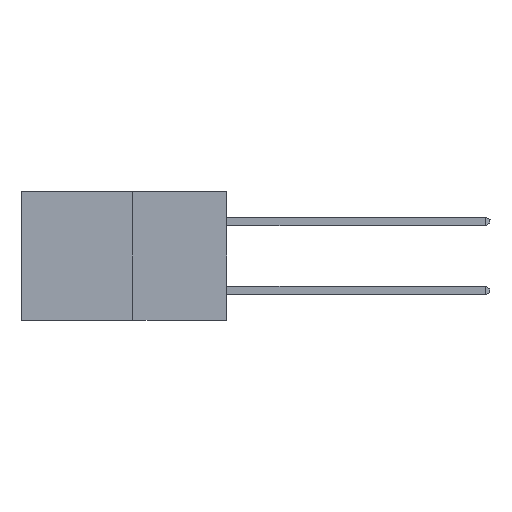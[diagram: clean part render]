
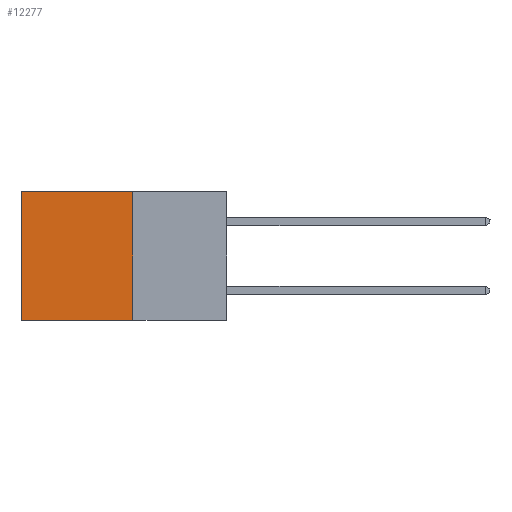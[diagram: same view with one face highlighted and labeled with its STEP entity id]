
A CAD part, left-side view. The second image highlights one B-rep face of the part: STEP entity #12277.
In plain terms, the highlighted planar face has unit normal (-1, 0, 0).
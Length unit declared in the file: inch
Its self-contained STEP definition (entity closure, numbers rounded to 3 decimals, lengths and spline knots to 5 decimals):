
#582 = EDGE_LOOP ( 'NONE', ( #15951, #666, #16527, #18513 ) ) ;
#633 = VERTEX_POINT ( 'NONE', #894 ) ;
#666 = ORIENTED_EDGE ( 'NONE', *, *, #5503, .F. ) ;
#894 = CARTESIAN_POINT ( 'NONE',  ( 0.277, 0.27, -0.37 ) ) ;
#1776 = EDGE_CURVE ( 'NONE', #5112, #1780, #6672, .T. ) ;
#1780 = VERTEX_POINT ( 'NONE', #5195 ) ;
#2743 = EDGE_CURVE ( 'NONE', #3079, #633, #12970, .T. ) ;
#3079 = VERTEX_POINT ( 'NONE', #8155 ) ;
#3580 = CARTESIAN_POINT ( 'NONE',  ( 0.277, 0.59, -0.37 ) ) ;
#3604 = DIRECTION ( 'NONE',  ( 0., 0., -1. ) ) ;
#5112 = VERTEX_POINT ( 'NONE', #13423 ) ;
#5195 = CARTESIAN_POINT ( 'NONE',  ( 0.277, 0.59, -0.37 ) ) ;
#5503 = EDGE_CURVE ( 'NONE', #633, #1780, #16423, .T. ) ;
#6672 = LINE ( 'NONE', #3580, #18489 ) ;
#7675 = CARTESIAN_POINT ( 'NONE',  ( 0.277, 0.27, -0.37 ) ) ;
#7895 = VECTOR ( 'NONE', #17598, 39.37008 ) ;
#8155 = CARTESIAN_POINT ( 'NONE',  ( 0.277, 0.27, 0. ) ) ;
#9320 = DIRECTION ( 'NONE',  ( 1., 0., 0. ) ) ;
#9651 = CARTESIAN_POINT ( 'NONE',  ( 0.277, 0.27, -0.37 ) ) ;
#10690 = LINE ( 'NONE', #20154, #19179 ) ;
#12277 = ADVANCED_FACE ( 'NONE', ( #13242 ), #17277, .F. ) ;
#12490 = VECTOR ( 'NONE', #15691, 39.37008 ) ;
#12956 = AXIS2_PLACEMENT_3D ( 'NONE', #7675, #9320, #20485 ) ;
#12970 = LINE ( 'NONE', #15427, #12490 ) ;
#13242 = FACE_OUTER_BOUND ( 'NONE', #582, .T. ) ;
#13423 = CARTESIAN_POINT ( 'NONE',  ( 0.277, 0.59, 0. ) ) ;
#13802 = DIRECTION ( 'NONE',  ( 0., 1., 0. ) ) ;
#14394 = EDGE_CURVE ( 'NONE', #3079, #5112, #10690, .T. ) ;
#15427 = CARTESIAN_POINT ( 'NONE',  ( 0.277, 0.27, -0.37 ) ) ;
#15691 = DIRECTION ( 'NONE',  ( 0., 0., -1. ) ) ;
#15951 = ORIENTED_EDGE ( 'NONE', *, *, #1776, .T. ) ;
#16423 = LINE ( 'NONE', #9651, #7895 ) ;
#16527 = ORIENTED_EDGE ( 'NONE', *, *, #2743, .F. ) ;
#17277 = PLANE ( 'NONE',  #12956 ) ;
#17598 = DIRECTION ( 'NONE',  ( 0., 1., 0. ) ) ;
#18489 = VECTOR ( 'NONE', #3604, 39.37008 ) ;
#18513 = ORIENTED_EDGE ( 'NONE', *, *, #14394, .T. ) ;
#19179 = VECTOR ( 'NONE', #13802, 39.37008 ) ;
#20154 = CARTESIAN_POINT ( 'NONE',  ( 0.277, 0.27, 0. ) ) ;
#20485 = DIRECTION ( 'NONE',  ( 0., 0., -1. ) ) ;
